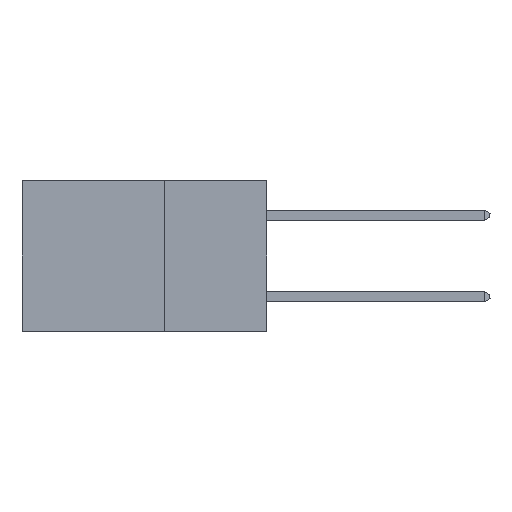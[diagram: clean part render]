
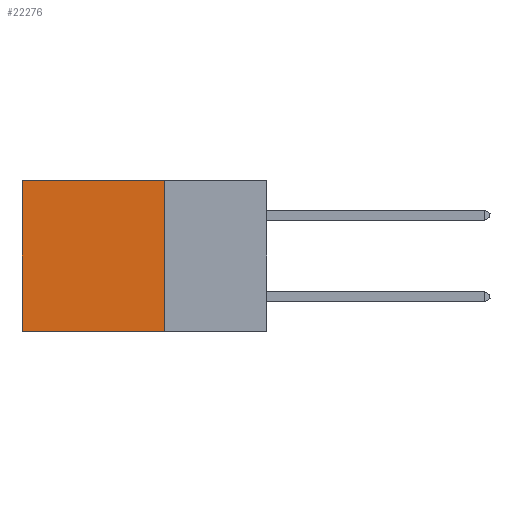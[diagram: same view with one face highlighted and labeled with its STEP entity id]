
A CAD part, left-side view. The second image highlights one B-rep face of the part: STEP entity #22276.
In plain terms, the highlighted planar face has unit normal (-1, 0, 0).
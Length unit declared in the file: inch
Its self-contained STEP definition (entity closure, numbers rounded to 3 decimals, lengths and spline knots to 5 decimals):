
#108 = LINE ( 'NONE', #1775, #2869 ) ;
#1775 = CARTESIAN_POINT ( 'NONE',  ( 0.2875, 0.25, 0. ) ) ;
#1794 = PLANE ( 'NONE',  #20222 ) ;
#2098 = ORIENTED_EDGE ( 'NONE', *, *, #2816, .T. ) ;
#2460 = DIRECTION ( 'NONE',  ( 0., 0., -1. ) ) ;
#2816 = EDGE_CURVE ( 'NONE', #23564, #6942, #22691, .T. ) ;
#2869 = VECTOR ( 'NONE', #3754, 39.37008 ) ;
#3754 = DIRECTION ( 'NONE',  ( 0., 0., -1. ) ) ;
#3855 = CARTESIAN_POINT ( 'NONE',  ( 0.2875, 0.25, -0.37 ) ) ;
#5790 = CARTESIAN_POINT ( 'NONE',  ( 0.2875, 0.25, -0.37 ) ) ;
#6015 = CARTESIAN_POINT ( 'NONE',  ( 0.2875, 0.25, 0. ) ) ;
#6942 = VERTEX_POINT ( 'NONE', #13852 ) ;
#7521 = EDGE_CURVE ( 'NONE', #23564, #24343, #108, .T. ) ;
#7764 = DIRECTION ( 'NONE',  ( 1., 0., 0. ) ) ;
#7879 = LINE ( 'NONE', #3855, #18486 ) ;
#8263 = ORIENTED_EDGE ( 'NONE', *, *, #7521, .F. ) ;
#9554 = CARTESIAN_POINT ( 'NONE',  ( 0.2875, 0.6, -0.37 ) ) ;
#9675 = EDGE_CURVE ( 'NONE', #24343, #12973, #7879, .T. ) ;
#10427 = CARTESIAN_POINT ( 'NONE',  ( 0.2875, 0.25, 0. ) ) ;
#11886 = CARTESIAN_POINT ( 'NONE',  ( 0.2875, 0.25, 0. ) ) ;
#12973 = VERTEX_POINT ( 'NONE', #9554 ) ;
#13852 = CARTESIAN_POINT ( 'NONE',  ( 0.2875, 0.6, 0. ) ) ;
#14297 = CARTESIAN_POINT ( 'NONE',  ( 0.2875, 0.6, 0. ) ) ;
#15508 = EDGE_CURVE ( 'NONE', #6942, #12973, #16703, .T. ) ;
#15793 = DIRECTION ( 'NONE',  ( 0., 0., -1. ) ) ;
#15988 = FACE_OUTER_BOUND ( 'NONE', #19615, .T. ) ;
#16399 = DIRECTION ( 'NONE',  ( 0., 1., 0. ) ) ;
#16703 = LINE ( 'NONE', #14297, #21338 ) ;
#18486 = VECTOR ( 'NONE', #23865, 39.37008 ) ;
#19295 = VECTOR ( 'NONE', #16399, 39.37008 ) ;
#19615 = EDGE_LOOP ( 'NONE', ( #23136, #21649, #8263, #2098 ) ) ;
#20222 = AXIS2_PLACEMENT_3D ( 'NONE', #6015, #7764, #15793 ) ;
#21338 = VECTOR ( 'NONE', #2460, 39.37008 ) ;
#21649 = ORIENTED_EDGE ( 'NONE', *, *, #9675, .F. ) ;
#22276 = ADVANCED_FACE ( 'NONE', ( #15988 ), #1794, .F. ) ;
#22691 = LINE ( 'NONE', #11886, #19295 ) ;
#23136 = ORIENTED_EDGE ( 'NONE', *, *, #15508, .T. ) ;
#23564 = VERTEX_POINT ( 'NONE', #10427 ) ;
#23865 = DIRECTION ( 'NONE',  ( 0., 1., 0. ) ) ;
#24343 = VERTEX_POINT ( 'NONE', #5790 ) ;
